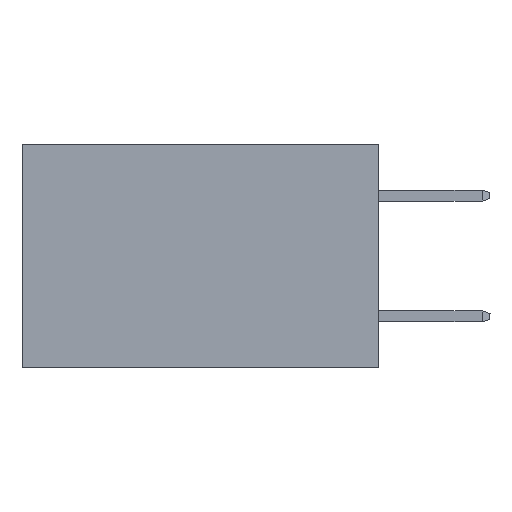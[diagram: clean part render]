
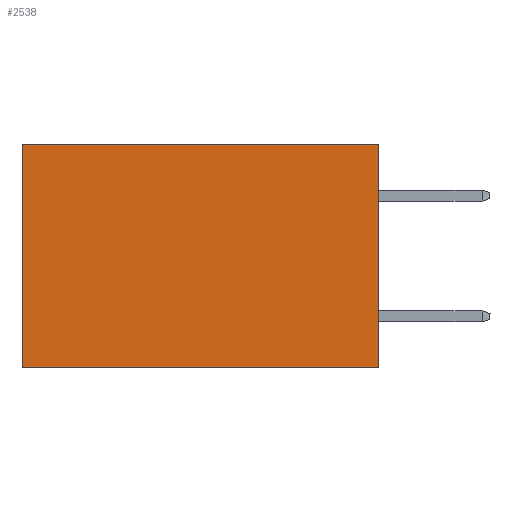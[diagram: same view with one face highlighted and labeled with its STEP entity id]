
A CAD part, left-side view. The second image highlights one B-rep face of the part: STEP entity #2538.
In plain terms, the highlighted planar face has unit normal (-1, 0, 0).
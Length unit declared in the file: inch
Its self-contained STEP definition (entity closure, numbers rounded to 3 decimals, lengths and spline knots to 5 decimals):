
#111 = CARTESIAN_POINT ( 'NONE',  ( 0.277, 0., -0.37 ) ) ;
#164 = EDGE_CURVE ( 'NONE', #26490, #31567, #7555, .T. ) ;
#1069 = CARTESIAN_POINT ( 'NONE',  ( 0.277, 0., 0. ) ) ;
#1281 = LINE ( 'NONE', #11829, #30596 ) ;
#1988 = EDGE_CURVE ( 'NONE', #18287, #2487, #22280, .T. ) ;
#2487 = VERTEX_POINT ( 'NONE', #27811 ) ;
#2538 = ADVANCED_FACE ( 'NONE', ( #6605 ), #27573, .F. ) ;
#2625 = LINE ( 'NONE', #12456, #15218 ) ;
#2799 = ORIENTED_EDGE ( 'NONE', *, *, #1988, .T. ) ;
#6605 = FACE_OUTER_BOUND ( 'NONE', #11690, .T. ) ;
#7555 = LINE ( 'NONE', #26923, #8333 ) ;
#8333 = VECTOR ( 'NONE', #29305, 39.37008 ) ;
#9788 = VECTOR ( 'NONE', #18199, 39.37008 ) ;
#11690 = EDGE_LOOP ( 'NONE', ( #22934, #31955, #15201, #2799 ) ) ;
#11829 = CARTESIAN_POINT ( 'NONE',  ( 0.277, 0.59, -0.37 ) ) ;
#12456 = CARTESIAN_POINT ( 'NONE',  ( 0.277, 0., -0.37 ) ) ;
#15201 = ORIENTED_EDGE ( 'NONE', *, *, #25993, .F. ) ;
#15218 = VECTOR ( 'NONE', #17456, 39.37008 ) ;
#16736 = AXIS2_PLACEMENT_3D ( 'NONE', #111, #19138, #17556 ) ;
#17456 = DIRECTION ( 'NONE',  ( 0., 0., -1. ) ) ;
#17556 = DIRECTION ( 'NONE',  ( 0., 0., -1. ) ) ;
#18199 = DIRECTION ( 'NONE',  ( 0., 1., 0. ) ) ;
#18238 = CARTESIAN_POINT ( 'NONE',  ( 0.277, 0., 0. ) ) ;
#18287 = VERTEX_POINT ( 'NONE', #1069 ) ;
#19138 = DIRECTION ( 'NONE',  ( 1., 0., 0. ) ) ;
#21453 = CARTESIAN_POINT ( 'NONE',  ( 0.277, 0., -0.37 ) ) ;
#22280 = LINE ( 'NONE', #18238, #9788 ) ;
#22934 = ORIENTED_EDGE ( 'NONE', *, *, #29717, .T. ) ;
#25940 = CARTESIAN_POINT ( 'NONE',  ( 0.277, 0.59, -0.37 ) ) ;
#25993 = EDGE_CURVE ( 'NONE', #18287, #26490, #2625, .T. ) ;
#26490 = VERTEX_POINT ( 'NONE', #21453 ) ;
#26811 = DIRECTION ( 'NONE',  ( 0., 0., -1. ) ) ;
#26923 = CARTESIAN_POINT ( 'NONE',  ( 0.277, 0., -0.37 ) ) ;
#27573 = PLANE ( 'NONE',  #16736 ) ;
#27811 = CARTESIAN_POINT ( 'NONE',  ( 0.277, 0.59, 0. ) ) ;
#29305 = DIRECTION ( 'NONE',  ( 0., 1., 0. ) ) ;
#29717 = EDGE_CURVE ( 'NONE', #2487, #31567, #1281, .T. ) ;
#30596 = VECTOR ( 'NONE', #26811, 39.37008 ) ;
#31567 = VERTEX_POINT ( 'NONE', #25940 ) ;
#31955 = ORIENTED_EDGE ( 'NONE', *, *, #164, .F. ) ;
